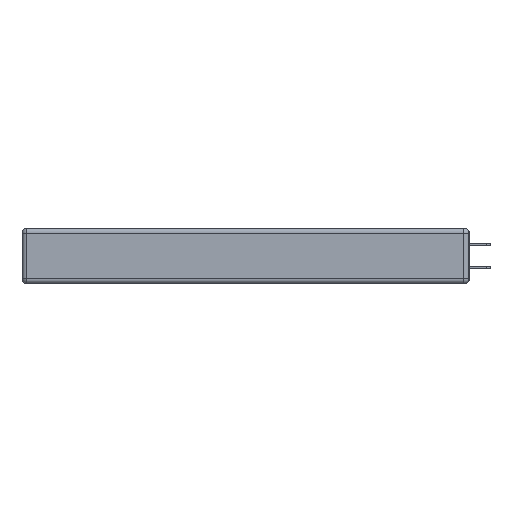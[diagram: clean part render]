
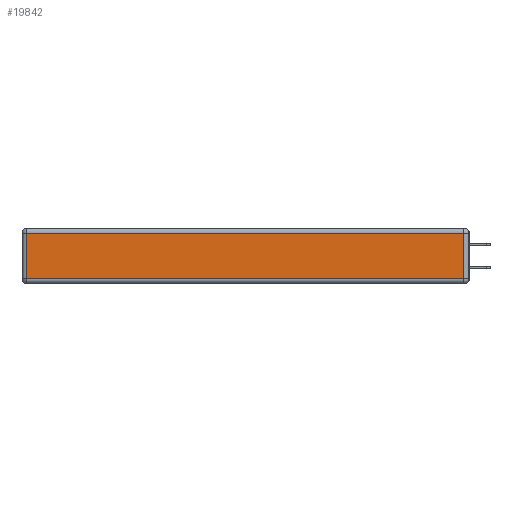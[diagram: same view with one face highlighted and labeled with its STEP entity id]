
A CAD part, left-side view. The second image highlights one B-rep face of the part: STEP entity #19842.
In plain terms, the highlighted planar face has unit normal (-1, 0, 0).
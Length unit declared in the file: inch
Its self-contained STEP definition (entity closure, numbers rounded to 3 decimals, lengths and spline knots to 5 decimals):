
#13 = CARTESIAN_POINT ( 'NONE',  ( 0., 2.72, -0.313 ) ) ;
#101 = CARTESIAN_POINT ( 'NONE',  ( 0., 0., -0.313 ) ) ;
#702 = ORIENTED_EDGE ( 'NONE', *, *, #19368, .T. ) ;
#844 = ORIENTED_EDGE ( 'NONE', *, *, #12600, .T. ) ;
#1519 = LINE ( 'NONE', #4477, #19953 ) ;
#1783 = VERTEX_POINT ( 'NONE', #13 ) ;
#1874 = VERTEX_POINT ( 'NONE', #3630 ) ;
#2186 = CARTESIAN_POINT ( 'NONE',  ( 0., 2.75, -0.03 ) ) ;
#2797 = VECTOR ( 'NONE', #11284, 39.37008 ) ;
#3630 = CARTESIAN_POINT ( 'NONE',  ( 0., 0.03, -0.313 ) ) ;
#3737 = FACE_OUTER_BOUND ( 'NONE', #17368, .T. ) ;
#4477 = CARTESIAN_POINT ( 'NONE',  ( 0., 2.72, -0.343 ) ) ;
#4670 = DIRECTION ( 'NONE',  ( -1., 0., 0. ) ) ;
#5775 = LINE ( 'NONE', #19673, #2797 ) ;
#7562 = LINE ( 'NONE', #101, #10505 ) ;
#7982 = LINE ( 'NONE', #2186, #12298 ) ;
#8021 = CARTESIAN_POINT ( 'NONE',  ( 0., 0., -0.343 ) ) ;
#8137 = DIRECTION ( 'NONE',  ( 0., 0., -1. ) ) ;
#9801 = VERTEX_POINT ( 'NONE', #19855 ) ;
#10505 = VECTOR ( 'NONE', #22179, 39.37008 ) ;
#10689 = CARTESIAN_POINT ( 'NONE',  ( 0., 2.72, -0.03 ) ) ;
#11284 = DIRECTION ( 'NONE',  ( 0., 0., 1. ) ) ;
#12298 = VECTOR ( 'NONE', #20956, 39.37008 ) ;
#12600 = EDGE_CURVE ( 'NONE', #1874, #9801, #5775, .T. ) ;
#14081 = EDGE_CURVE ( 'NONE', #1783, #1874, #7562, .T. ) ;
#16386 = PLANE ( 'NONE',  #21233 ) ;
#17291 = ORIENTED_EDGE ( 'NONE', *, *, #14081, .T. ) ;
#17368 = EDGE_LOOP ( 'NONE', ( #17291, #844, #702, #19549 ) ) ;
#17627 = VERTEX_POINT ( 'NONE', #10689 ) ;
#19368 = EDGE_CURVE ( 'NONE', #9801, #17627, #7982, .T. ) ;
#19549 = ORIENTED_EDGE ( 'NONE', *, *, #21210, .T. ) ;
#19673 = CARTESIAN_POINT ( 'NONE',  ( 0., 0.03, -0.343 ) ) ;
#19842 = ADVANCED_FACE ( 'NONE', ( #3737 ), #16386, .T. ) ;
#19855 = CARTESIAN_POINT ( 'NONE',  ( 0., 0.03, -0.03 ) ) ;
#19953 = VECTOR ( 'NONE', #8137, 39.37008 ) ;
#19981 = DIRECTION ( 'NONE',  ( 0., 0., 1. ) ) ;
#20956 = DIRECTION ( 'NONE',  ( 0., 1., 0. ) ) ;
#21210 = EDGE_CURVE ( 'NONE', #17627, #1783, #1519, .T. ) ;
#21233 = AXIS2_PLACEMENT_3D ( 'NONE', #8021, #4670, #19981 ) ;
#22179 = DIRECTION ( 'NONE',  ( 0., -1., 0. ) ) ;
